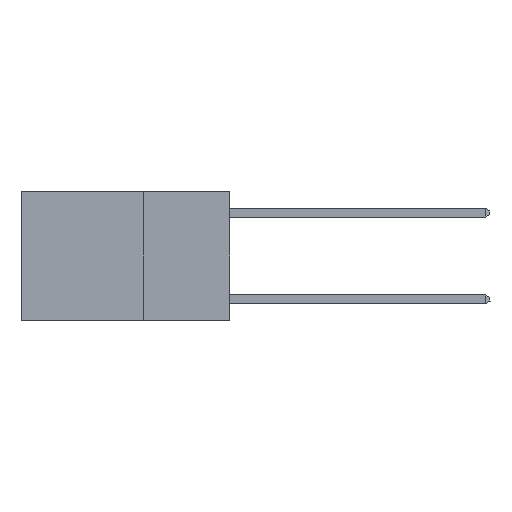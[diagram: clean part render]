
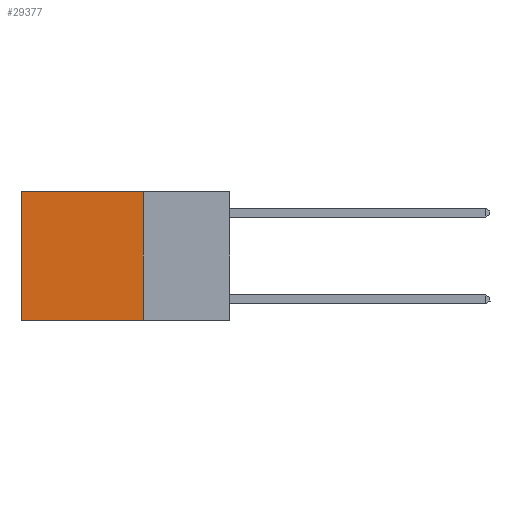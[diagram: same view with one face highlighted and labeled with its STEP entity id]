
A CAD part, left-side view. The second image highlights one B-rep face of the part: STEP entity #29377.
In plain terms, the highlighted planar face has unit normal (-1, 0, 0).
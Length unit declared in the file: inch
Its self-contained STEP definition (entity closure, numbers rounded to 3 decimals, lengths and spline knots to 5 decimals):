
#768 = DIRECTION ( 'NONE',  ( 0., 1., 0. ) ) ;
#1342 = VERTEX_POINT ( 'NONE', #8962 ) ;
#1416 = DIRECTION ( 'NONE',  ( 1., 0., 0. ) ) ;
#4305 = CARTESIAN_POINT ( 'NONE',  ( 0.2625, 0.6, 0. ) ) ;
#4498 = CARTESIAN_POINT ( 'NONE',  ( 0.2625, 0.6, -0.37 ) ) ;
#5261 = VECTOR ( 'NONE', #21352, 39.37008 ) ;
#5376 = VECTOR ( 'NONE', #21763, 39.37008 ) ;
#5655 = AXIS2_PLACEMENT_3D ( 'NONE', #28877, #1416, #17540 ) ;
#5900 = LINE ( 'NONE', #8738, #22771 ) ;
#6264 = LINE ( 'NONE', #16925, #23871 ) ;
#8738 = CARTESIAN_POINT ( 'NONE',  ( 0.2625, 0.25, 0. ) ) ;
#8962 = CARTESIAN_POINT ( 'NONE',  ( 0.2625, 0.25, 0. ) ) ;
#9043 = FACE_OUTER_BOUND ( 'NONE', #14755, .T. ) ;
#9044 = EDGE_CURVE ( 'NONE', #18637, #9513, #6264, .T. ) ;
#9513 = VERTEX_POINT ( 'NONE', #4498 ) ;
#11593 = EDGE_CURVE ( 'NONE', #15530, #9513, #19753, .T. ) ;
#12877 = PLANE ( 'NONE',  #5655 ) ;
#14755 = EDGE_LOOP ( 'NONE', ( #15059, #15420, #15849, #16439 ) ) ;
#15059 = ORIENTED_EDGE ( 'NONE', *, *, #11593, .T. ) ;
#15420 = ORIENTED_EDGE ( 'NONE', *, *, #9044, .F. ) ;
#15530 = VERTEX_POINT ( 'NONE', #4305 ) ;
#15849 = ORIENTED_EDGE ( 'NONE', *, *, #28872, .F. ) ;
#16439 = ORIENTED_EDGE ( 'NONE', *, *, #24288, .T. ) ;
#16925 = CARTESIAN_POINT ( 'NONE',  ( 0.2625, 0.25, -0.37 ) ) ;
#17514 = LINE ( 'NONE', #23567, #5261 ) ;
#17540 = DIRECTION ( 'NONE',  ( 0., 0., -1. ) ) ;
#18637 = VERTEX_POINT ( 'NONE', #29179 ) ;
#19753 = LINE ( 'NONE', #26272, #5376 ) ;
#20317 = DIRECTION ( 'NONE',  ( 0., 0., -1. ) ) ;
#21352 = DIRECTION ( 'NONE',  ( 0., 1., 0. ) ) ;
#21763 = DIRECTION ( 'NONE',  ( 0., 0., -1. ) ) ;
#22771 = VECTOR ( 'NONE', #20317, 39.37008 ) ;
#23567 = CARTESIAN_POINT ( 'NONE',  ( 0.2625, 0.25, 0. ) ) ;
#23871 = VECTOR ( 'NONE', #768, 39.37008 ) ;
#24288 = EDGE_CURVE ( 'NONE', #1342, #15530, #17514, .T. ) ;
#26272 = CARTESIAN_POINT ( 'NONE',  ( 0.2625, 0.6, 0. ) ) ;
#28872 = EDGE_CURVE ( 'NONE', #1342, #18637, #5900, .T. ) ;
#28877 = CARTESIAN_POINT ( 'NONE',  ( 0.2625, 0.25, 0. ) ) ;
#29179 = CARTESIAN_POINT ( 'NONE',  ( 0.2625, 0.25, -0.37 ) ) ;
#29377 = ADVANCED_FACE ( 'NONE', ( #9043 ), #12877, .F. ) ;
